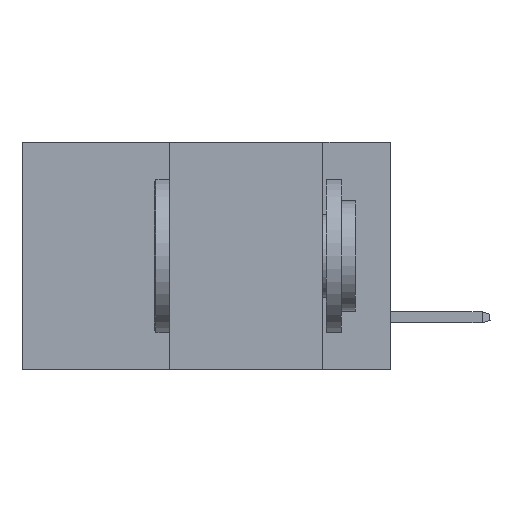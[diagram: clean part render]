
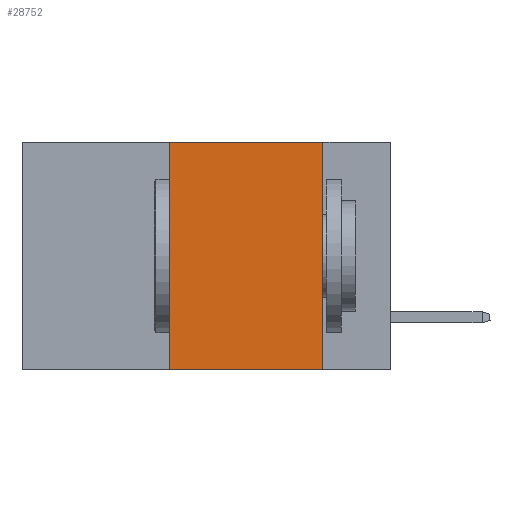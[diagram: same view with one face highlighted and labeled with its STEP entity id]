
A CAD part, left-side view. The second image highlights one B-rep face of the part: STEP entity #28752.
In plain terms, the highlighted planar face has unit normal (-1, 0, 0).
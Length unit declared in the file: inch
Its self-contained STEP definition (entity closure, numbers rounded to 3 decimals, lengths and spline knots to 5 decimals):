
#343 = LINE ( 'NONE', #23231, #24878 ) ;
#669 = LINE ( 'NONE', #10961, #33724 ) ;
#941 = DIRECTION ( 'NONE',  ( 1., 0., 0. ) ) ;
#2108 = CARTESIAN_POINT ( 'NONE',  ( 0., 0.36, 0. ) ) ;
#3699 = VERTEX_POINT ( 'NONE', #6975 ) ;
#6604 = EDGE_CURVE ( 'NONE', #8474, #3699, #343, .T. ) ;
#6975 = CARTESIAN_POINT ( 'NONE',  ( 0., 0.11, -0.37 ) ) ;
#8115 = CARTESIAN_POINT ( 'NONE',  ( 0., 0.36, 0. ) ) ;
#8474 = VERTEX_POINT ( 'NONE', #10830 ) ;
#9532 = PLANE ( 'NONE',  #22469 ) ;
#10489 = EDGE_CURVE ( 'NONE', #13817, #3699, #20987, .T. ) ;
#10830 = CARTESIAN_POINT ( 'NONE',  ( 0., 0.36, -0.37 ) ) ;
#10961 = CARTESIAN_POINT ( 'NONE',  ( 0., 0.6, 0. ) ) ;
#13817 = VERTEX_POINT ( 'NONE', #27822 ) ;
#14242 = ORIENTED_EDGE ( 'NONE', *, *, #10489, .F. ) ;
#16703 = VERTEX_POINT ( 'NONE', #8115 ) ;
#17467 = EDGE_CURVE ( 'NONE', #16703, #13817, #669, .T. ) ;
#17607 = VECTOR ( 'NONE', #26884, 39.37008 ) ;
#19924 = ORIENTED_EDGE ( 'NONE', *, *, #6604, .T. ) ;
#20987 = LINE ( 'NONE', #32534, #24867 ) ;
#22469 = AXIS2_PLACEMENT_3D ( 'NONE', #26048, #941, #25810 ) ;
#23231 = CARTESIAN_POINT ( 'NONE',  ( 0., 0.6, -0.37 ) ) ;
#23369 = ORIENTED_EDGE ( 'NONE', *, *, #17467, .F. ) ;
#23412 = EDGE_LOOP ( 'NONE', ( #14242, #23369, #31781, #19924 ) ) ;
#24023 = EDGE_CURVE ( 'NONE', #8474, #16703, #24931, .T. ) ;
#24867 = VECTOR ( 'NONE', #32645, 39.37008 ) ;
#24878 = VECTOR ( 'NONE', #33870, 39.37008 ) ;
#24931 = LINE ( 'NONE', #2108, #17607 ) ;
#25810 = DIRECTION ( 'NONE',  ( 0., 0., -1. ) ) ;
#26048 = CARTESIAN_POINT ( 'NONE',  ( 0., 0.6, 0. ) ) ;
#26884 = DIRECTION ( 'NONE',  ( 0., 0., 1. ) ) ;
#27803 = DIRECTION ( 'NONE',  ( 0., -1., 0. ) ) ;
#27822 = CARTESIAN_POINT ( 'NONE',  ( 0., 0.11, 0. ) ) ;
#28752 = ADVANCED_FACE ( 'NONE', ( #35011 ), #9532, .F. ) ;
#31781 = ORIENTED_EDGE ( 'NONE', *, *, #24023, .F. ) ;
#32534 = CARTESIAN_POINT ( 'NONE',  ( 0., 0.11, 0. ) ) ;
#32645 = DIRECTION ( 'NONE',  ( 0., 0., -1. ) ) ;
#33724 = VECTOR ( 'NONE', #27803, 39.37008 ) ;
#33870 = DIRECTION ( 'NONE',  ( 0., -1., 0. ) ) ;
#35011 = FACE_OUTER_BOUND ( 'NONE', #23412, .T. ) ;
